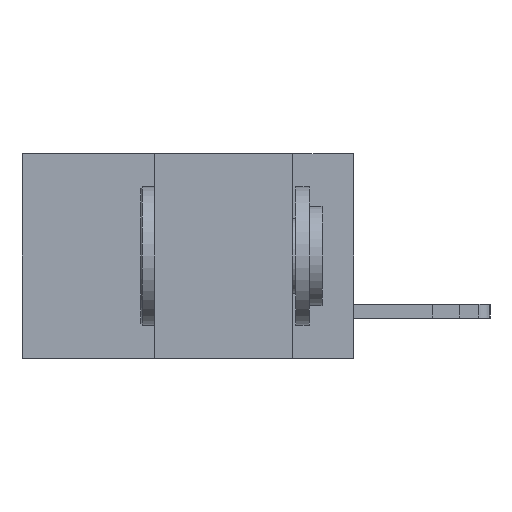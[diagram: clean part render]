
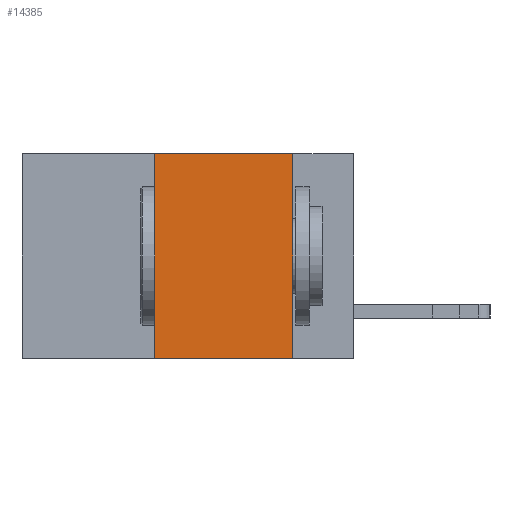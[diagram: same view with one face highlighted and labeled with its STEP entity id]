
A CAD part, left-side view. The second image highlights one B-rep face of the part: STEP entity #14385.
In plain terms, the highlighted planar face has unit normal (-1, 0, 0).
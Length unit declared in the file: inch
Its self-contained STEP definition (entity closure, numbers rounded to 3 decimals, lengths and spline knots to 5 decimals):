
#450 = EDGE_CURVE ( 'NONE', #11929, #9031, #15568, .T. ) ;
#1225 = DIRECTION ( 'NONE',  ( 0., 0., -1. ) ) ;
#2337 = PLANE ( 'NONE',  #11262 ) ;
#3789 = FACE_OUTER_BOUND ( 'NONE', #12265, .T. ) ;
#4270 = ORIENTED_EDGE ( 'NONE', *, *, #450, .F. ) ;
#4649 = DIRECTION ( 'NONE',  ( 0., 0., -1. ) ) ;
#4952 = ORIENTED_EDGE ( 'NONE', *, *, #11530, .F. ) ;
#6393 = EDGE_CURVE ( 'NONE', #11929, #9377, #14375, .T. ) ;
#6756 = VECTOR ( 'NONE', #13247, 39.37008 ) ;
#6855 = VECTOR ( 'NONE', #15471, 39.37008 ) ;
#6900 = ORIENTED_EDGE ( 'NONE', *, *, #6393, .T. ) ;
#8188 = CARTESIAN_POINT ( 'NONE',  ( 0., 0.36, -0.37 ) ) ;
#8888 = LINE ( 'NONE', #14164, #6855 ) ;
#9031 = VERTEX_POINT ( 'NONE', #9381 ) ;
#9377 = VERTEX_POINT ( 'NONE', #15352 ) ;
#9381 = CARTESIAN_POINT ( 'NONE',  ( 0., 0.36, 0. ) ) ;
#9891 = ORIENTED_EDGE ( 'NONE', *, *, #14737, .F. ) ;
#10176 = CARTESIAN_POINT ( 'NONE',  ( 0., 0.6, 0. ) ) ;
#10858 = CARTESIAN_POINT ( 'NONE',  ( 0., 0.11, 0. ) ) ;
#11262 = AXIS2_PLACEMENT_3D ( 'NONE', #10176, #11390, #1225 ) ;
#11390 = DIRECTION ( 'NONE',  ( 1., 0., 0. ) ) ;
#11505 = VERTEX_POINT ( 'NONE', #11701 ) ;
#11530 = EDGE_CURVE ( 'NONE', #9031, #11505, #8888, .T. ) ;
#11572 = DIRECTION ( 'NONE',  ( 0., -1., 0. ) ) ;
#11627 = VECTOR ( 'NONE', #11572, 39.37008 ) ;
#11701 = CARTESIAN_POINT ( 'NONE',  ( 0., 0.11, 0. ) ) ;
#11929 = VERTEX_POINT ( 'NONE', #8188 ) ;
#12265 = EDGE_LOOP ( 'NONE', ( #9891, #4952, #4270, #6900 ) ) ;
#12766 = CARTESIAN_POINT ( 'NONE',  ( 0., 0.6, -0.37 ) ) ;
#13159 = CARTESIAN_POINT ( 'NONE',  ( 0., 0.36, 0. ) ) ;
#13247 = DIRECTION ( 'NONE',  ( 0., 0., 1. ) ) ;
#14164 = CARTESIAN_POINT ( 'NONE',  ( 0., 0.6, 0. ) ) ;
#14375 = LINE ( 'NONE', #12766, #11627 ) ;
#14385 = ADVANCED_FACE ( 'NONE', ( #3789 ), #2337, .F. ) ;
#14737 = EDGE_CURVE ( 'NONE', #11505, #9377, #16076, .T. ) ;
#15352 = CARTESIAN_POINT ( 'NONE',  ( 0., 0.11, -0.37 ) ) ;
#15471 = DIRECTION ( 'NONE',  ( 0., -1., 0. ) ) ;
#15568 = LINE ( 'NONE', #13159, #6756 ) ;
#16076 = LINE ( 'NONE', #10858, #16738 ) ;
#16738 = VECTOR ( 'NONE', #4649, 39.37008 ) ;
